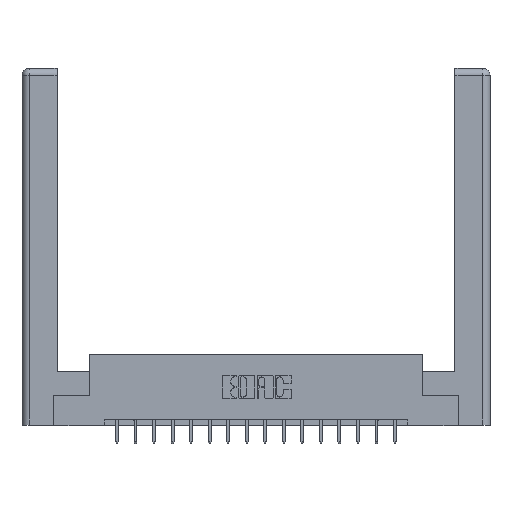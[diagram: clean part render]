
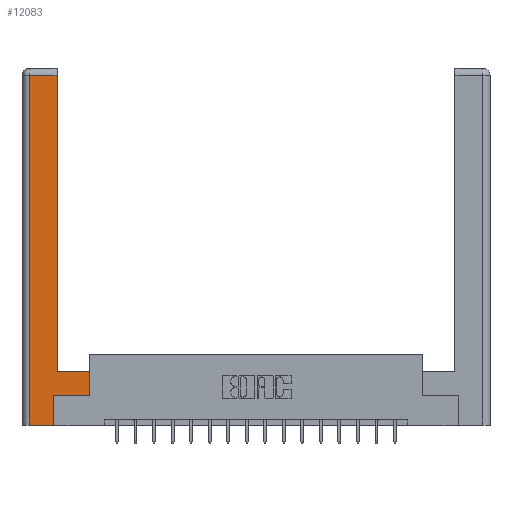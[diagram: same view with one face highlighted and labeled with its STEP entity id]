
A CAD part, top view. The second image highlights one B-rep face of the part: STEP entity #12083.
In plain terms, the highlighted planar face has unit normal (0, 0, 1).
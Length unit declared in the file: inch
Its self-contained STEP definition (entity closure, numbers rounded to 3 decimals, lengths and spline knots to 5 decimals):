
#124 = CARTESIAN_POINT ( 'NONE',  ( 0.565, 0.45, 0. ) ) ;
#324 = VERTEX_POINT ( 'NONE', #14201 ) ;
#691 = CARTESIAN_POINT ( 'NONE',  ( 0.265, 0.245, 0. ) ) ;
#845 = EDGE_LOOP ( 'NONE', ( #15050, #11539, #3509, #15711, #3374, #18209, #1299, #3696 ) ) ;
#1041 = CARTESIAN_POINT ( 'NONE',  ( 0.0615, 0., 0. ) ) ;
#1053 = DIRECTION ( 'NONE',  ( 0., 0., -1. ) ) ;
#1219 = CARTESIAN_POINT ( 'NONE',  ( 0.265, 0., 0. ) ) ;
#1299 = ORIENTED_EDGE ( 'NONE', *, *, #12513, .T. ) ;
#1459 = DIRECTION ( 'NONE',  ( -1., 0., 0. ) ) ;
#2628 = VERTEX_POINT ( 'NONE', #6372 ) ;
#2954 = VERTEX_POINT ( 'NONE', #1219 ) ;
#2986 = VERTEX_POINT ( 'NONE', #7951 ) ;
#3288 = LINE ( 'NONE', #11494, #6183 ) ;
#3374 = ORIENTED_EDGE ( 'NONE', *, *, #12821, .T. ) ;
#3509 = ORIENTED_EDGE ( 'NONE', *, *, #17390, .T. ) ;
#3696 = ORIENTED_EDGE ( 'NONE', *, *, #16818, .T. ) ;
#3821 = DIRECTION ( 'NONE',  ( -1., 0., 0. ) ) ;
#4223 = VECTOR ( 'NONE', #4524, 39.37008 ) ;
#4524 = DIRECTION ( 'NONE',  ( 0., 1., 0. ) ) ;
#4631 = LINE ( 'NONE', #5892, #9100 ) ;
#4750 = CARTESIAN_POINT ( 'NONE',  ( 0.565, 0.245, 0. ) ) ;
#4777 = EDGE_CURVE ( 'NONE', #2986, #12067, #4631, .T. ) ;
#5212 = LINE ( 'NONE', #8702, #9464 ) ;
#5316 = VECTOR ( 'NONE', #12405, 39.37008 ) ;
#5581 = CARTESIAN_POINT ( 'NONE',  ( 0.265, 0., 0. ) ) ;
#5710 = DIRECTION ( 'NONE',  ( 0., 1., 0. ) ) ;
#5800 = VERTEX_POINT ( 'NONE', #16671 ) ;
#5892 = CARTESIAN_POINT ( 'NONE',  ( 0.0615, 2.94, 0. ) ) ;
#5893 = FACE_OUTER_BOUND ( 'NONE', #845, .T. ) ;
#6177 = DIRECTION ( 'NONE',  ( 1., 0., 0. ) ) ;
#6183 = VECTOR ( 'NONE', #8698, 39.37008 ) ;
#6222 = LINE ( 'NONE', #16516, #5316 ) ;
#6372 = CARTESIAN_POINT ( 'NONE',  ( 0.565, 0.245, 0. ) ) ;
#7231 = EDGE_CURVE ( 'NONE', #324, #2628, #15181, .T. ) ;
#7951 = CARTESIAN_POINT ( 'NONE',  ( 0.295, 2.94, 0. ) ) ;
#8384 = DIRECTION ( 'NONE',  ( 1., 0., 0. ) ) ;
#8698 = DIRECTION ( 'NONE',  ( 0., -1., 0. ) ) ;
#8702 = CARTESIAN_POINT ( 'NONE',  ( 0.565, 0.45, 0. ) ) ;
#9100 = VECTOR ( 'NONE', #1459, 39.37008 ) ;
#9143 = VECTOR ( 'NONE', #8384, 39.37008 ) ;
#9464 = VECTOR ( 'NONE', #5710, 39.37008 ) ;
#9675 = VECTOR ( 'NONE', #14939, 39.37008 ) ;
#9678 = CARTESIAN_POINT ( 'NONE',  ( 0.0615, 2.94, 0. ) ) ;
#9743 = EDGE_CURVE ( 'NONE', #5800, #2986, #12913, .T. ) ;
#10675 = LINE ( 'NONE', #5581, #9143 ) ;
#10943 = AXIS2_PLACEMENT_3D ( 'NONE', #11145, #1053, #3821 ) ;
#11145 = CARTESIAN_POINT ( 'NONE',  ( 0., 0., 0. ) ) ;
#11326 = VERTEX_POINT ( 'NONE', #124 ) ;
#11494 = CARTESIAN_POINT ( 'NONE',  ( 0.0615, 0., 0. ) ) ;
#11539 = ORIENTED_EDGE ( 'NONE', *, *, #4777, .T. ) ;
#12067 = VERTEX_POINT ( 'NONE', #9678 ) ;
#12083 = ADVANCED_FACE ( 'NONE', ( #5893 ), #15427, .F. ) ;
#12405 = DIRECTION ( 'NONE',  ( -1., 0., 0. ) ) ;
#12513 = EDGE_CURVE ( 'NONE', #2628, #11326, #5212, .T. ) ;
#12821 = EDGE_CURVE ( 'NONE', #2954, #324, #14534, .T. ) ;
#12913 = LINE ( 'NONE', #14572, #4223 ) ;
#13602 = VECTOR ( 'NONE', #6177, 39.37008 ) ;
#14201 = CARTESIAN_POINT ( 'NONE',  ( 0.265, 0.245, 0. ) ) ;
#14534 = LINE ( 'NONE', #691, #9675 ) ;
#14572 = CARTESIAN_POINT ( 'NONE',  ( 0.295, 3., 0. ) ) ;
#14770 = EDGE_CURVE ( 'NONE', #17812, #2954, #10675, .T. ) ;
#14939 = DIRECTION ( 'NONE',  ( 0., 1., 0. ) ) ;
#15050 = ORIENTED_EDGE ( 'NONE', *, *, #9743, .T. ) ;
#15181 = LINE ( 'NONE', #4750, #13602 ) ;
#15427 = PLANE ( 'NONE',  #10943 ) ;
#15711 = ORIENTED_EDGE ( 'NONE', *, *, #14770, .T. ) ;
#16516 = CARTESIAN_POINT ( 'NONE',  ( 0.295, 0.45, 0. ) ) ;
#16671 = CARTESIAN_POINT ( 'NONE',  ( 0.295, 0.45, 0. ) ) ;
#16818 = EDGE_CURVE ( 'NONE', #11326, #5800, #6222, .T. ) ;
#17390 = EDGE_CURVE ( 'NONE', #12067, #17812, #3288, .T. ) ;
#17812 = VERTEX_POINT ( 'NONE', #1041 ) ;
#18209 = ORIENTED_EDGE ( 'NONE', *, *, #7231, .T. ) ;
